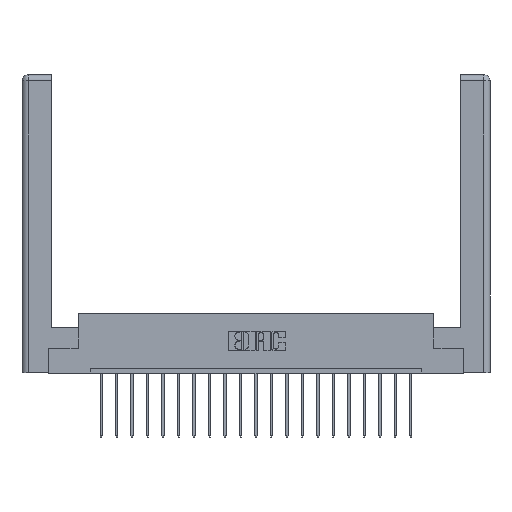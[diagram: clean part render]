
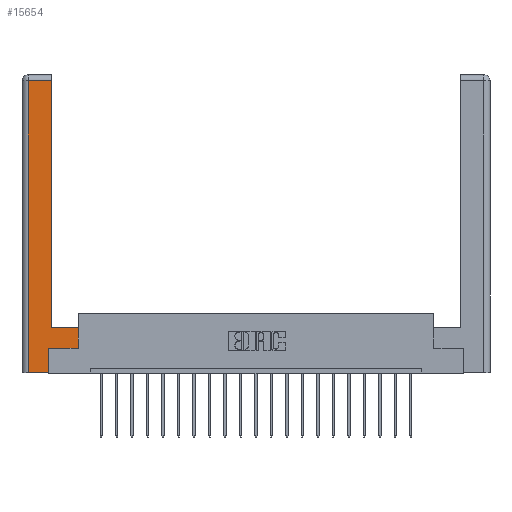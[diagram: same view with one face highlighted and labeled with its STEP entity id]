
A CAD part, top view. The second image highlights one B-rep face of the part: STEP entity #15654.
In plain terms, the highlighted planar face has unit normal (0, 0, 1).
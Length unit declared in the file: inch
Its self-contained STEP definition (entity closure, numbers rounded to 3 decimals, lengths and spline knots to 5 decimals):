
#435 = CARTESIAN_POINT ( 'NONE',  ( 0.265, 0., 0. ) ) ;
#841 = CARTESIAN_POINT ( 'NONE',  ( 0.565, 0.45, 0. ) ) ;
#1175 = DIRECTION ( 'NONE',  ( 0., -1., 0. ) ) ;
#1379 = VECTOR ( 'NONE', #20119, 39.37008 ) ;
#1572 = DIRECTION ( 'NONE',  ( 1., 0., 0. ) ) ;
#1579 = ORIENTED_EDGE ( 'NONE', *, *, #19059, .T. ) ;
#1633 = VECTOR ( 'NONE', #9279, 39.37008 ) ;
#2141 = LINE ( 'NONE', #6592, #17363 ) ;
#2590 = VECTOR ( 'NONE', #10050, 39.37008 ) ;
#2638 = VECTOR ( 'NONE', #19808, 39.37008 ) ;
#3367 = VECTOR ( 'NONE', #1572, 39.37008 ) ;
#3501 = EDGE_CURVE ( 'NONE', #12273, #9079, #7134, .T. ) ;
#3755 = ORIENTED_EDGE ( 'NONE', *, *, #10885, .T. ) ;
#4130 = CARTESIAN_POINT ( 'NONE',  ( 0.295, 0.45, 0. ) ) ;
#4370 = VERTEX_POINT ( 'NONE', #435 ) ;
#5507 = EDGE_CURVE ( 'NONE', #19573, #4370, #19627, .T. ) ;
#5620 = CARTESIAN_POINT ( 'NONE',  ( 0., 0., 0. ) ) ;
#5677 = CARTESIAN_POINT ( 'NONE',  ( 0.295, 2.94, 0. ) ) ;
#6592 = CARTESIAN_POINT ( 'NONE',  ( 0.295, 0.45, 0. ) ) ;
#7134 = LINE ( 'NONE', #9975, #2590 ) ;
#7232 = DIRECTION ( 'NONE',  ( 0., 0., -1. ) ) ;
#7552 = VECTOR ( 'NONE', #1175, 39.37008 ) ;
#7866 = VERTEX_POINT ( 'NONE', #16294 ) ;
#7948 = CARTESIAN_POINT ( 'NONE',  ( 0.565, 0.245, 0. ) ) ;
#8476 = ORIENTED_EDGE ( 'NONE', *, *, #19526, .T. ) ;
#8942 = CARTESIAN_POINT ( 'NONE',  ( 0.565, 0.245, 0. ) ) ;
#9079 = VERTEX_POINT ( 'NONE', #19931 ) ;
#9279 = DIRECTION ( 'NONE',  ( 0., 1., 0. ) ) ;
#9397 = CARTESIAN_POINT ( 'NONE',  ( 0.265, 0., 0. ) ) ;
#9444 = LINE ( 'NONE', #7948, #3367 ) ;
#9639 = VERTEX_POINT ( 'NONE', #8942 ) ;
#9745 = LINE ( 'NONE', #841, #1379 ) ;
#9916 = VECTOR ( 'NONE', #19711, 39.37008 ) ;
#9975 = CARTESIAN_POINT ( 'NONE',  ( 0.0615, 2.94, 0. ) ) ;
#10050 = DIRECTION ( 'NONE',  ( -1., 0., 0. ) ) ;
#10300 = EDGE_CURVE ( 'NONE', #15837, #18892, #2141, .T. ) ;
#10858 = CARTESIAN_POINT ( 'NONE',  ( 0.0615, 0., 0. ) ) ;
#10885 = EDGE_CURVE ( 'NONE', #9079, #19573, #12617, .T. ) ;
#10937 = LINE ( 'NONE', #11461, #9916 ) ;
#11461 = CARTESIAN_POINT ( 'NONE',  ( 0.265, 0.245, 0. ) ) ;
#12273 = VERTEX_POINT ( 'NONE', #5677 ) ;
#12453 = CARTESIAN_POINT ( 'NONE',  ( 0.565, 0.45, 0. ) ) ;
#12617 = LINE ( 'NONE', #10858, #7552 ) ;
#13146 = ORIENTED_EDGE ( 'NONE', *, *, #3501, .T. ) ;
#13780 = EDGE_CURVE ( 'NONE', #7866, #9639, #9444, .T. ) ;
#15447 = DIRECTION ( 'NONE',  ( -1., 0., 0. ) ) ;
#15654 = ADVANCED_FACE ( 'NONE', ( #19765 ), #18669, .F. ) ;
#15655 = CARTESIAN_POINT ( 'NONE',  ( 0.295, 3., 0. ) ) ;
#15837 = VERTEX_POINT ( 'NONE', #12453 ) ;
#16294 = CARTESIAN_POINT ( 'NONE',  ( 0.265, 0.245, 0. ) ) ;
#16610 = AXIS2_PLACEMENT_3D ( 'NONE', #5620, #7232, #15447 ) ;
#16663 = CARTESIAN_POINT ( 'NONE',  ( 0.0615, 0., 0. ) ) ;
#17363 = VECTOR ( 'NONE', #19568, 39.37008 ) ;
#17408 = EDGE_LOOP ( 'NONE', ( #8476, #13146, #3755, #18272, #1579, #19338, #20448, #19922 ) ) ;
#17992 = EDGE_CURVE ( 'NONE', #9639, #15837, #9745, .T. ) ;
#18272 = ORIENTED_EDGE ( 'NONE', *, *, #5507, .T. ) ;
#18669 = PLANE ( 'NONE',  #16610 ) ;
#18892 = VERTEX_POINT ( 'NONE', #4130 ) ;
#18907 = LINE ( 'NONE', #15655, #1633 ) ;
#19059 = EDGE_CURVE ( 'NONE', #4370, #7866, #10937, .T. ) ;
#19338 = ORIENTED_EDGE ( 'NONE', *, *, #13780, .T. ) ;
#19526 = EDGE_CURVE ( 'NONE', #18892, #12273, #18907, .T. ) ;
#19568 = DIRECTION ( 'NONE',  ( -1., 0., 0. ) ) ;
#19573 = VERTEX_POINT ( 'NONE', #16663 ) ;
#19627 = LINE ( 'NONE', #9397, #2638 ) ;
#19711 = DIRECTION ( 'NONE',  ( 0., 1., 0. ) ) ;
#19765 = FACE_OUTER_BOUND ( 'NONE', #17408, .T. ) ;
#19808 = DIRECTION ( 'NONE',  ( 1., 0., 0. ) ) ;
#19922 = ORIENTED_EDGE ( 'NONE', *, *, #10300, .T. ) ;
#19931 = CARTESIAN_POINT ( 'NONE',  ( 0.0615, 2.94, 0. ) ) ;
#20119 = DIRECTION ( 'NONE',  ( 0., 1., 0. ) ) ;
#20448 = ORIENTED_EDGE ( 'NONE', *, *, #17992, .T. ) ;
